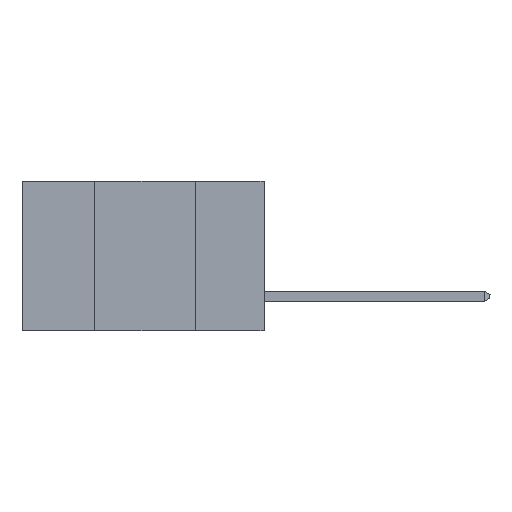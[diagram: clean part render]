
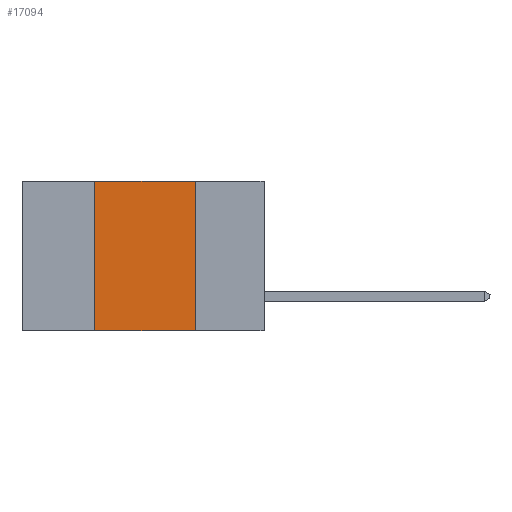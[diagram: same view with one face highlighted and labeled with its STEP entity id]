
A CAD part, left-side view. The second image highlights one B-rep face of the part: STEP entity #17094.
In plain terms, the highlighted planar face has unit normal (-1, 0, 0).
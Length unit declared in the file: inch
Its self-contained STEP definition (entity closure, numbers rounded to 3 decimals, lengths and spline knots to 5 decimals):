
#972 = VERTEX_POINT ( 'NONE', #8678 ) ;
#1638 = DIRECTION ( 'NONE',  ( 0., 0., -1. ) ) ;
#3787 = VECTOR ( 'NONE', #4854, 39.37008 ) ;
#4854 = DIRECTION ( 'NONE',  ( 0., -1., 0. ) ) ;
#5273 = EDGE_LOOP ( 'NONE', ( #5302, #8342, #9848, #22234 ) ) ;
#5302 = ORIENTED_EDGE ( 'NONE', *, *, #13556, .F. ) ;
#5391 = LINE ( 'NONE', #8872, #3787 ) ;
#5508 = LINE ( 'NONE', #22607, #10928 ) ;
#5584 = AXIS2_PLACEMENT_3D ( 'NONE', #26096, #13872, #1638 ) ;
#5923 = EDGE_CURVE ( 'NONE', #19945, #9236, #24880, .T. ) ;
#6390 = DIRECTION ( 'NONE',  ( 0., 0., 1. ) ) ;
#6781 = CARTESIAN_POINT ( 'NONE',  ( 0., 0.6, -0.37 ) ) ;
#8342 = ORIENTED_EDGE ( 'NONE', *, *, #11159, .F. ) ;
#8678 = CARTESIAN_POINT ( 'NONE',  ( 0., 0.42, 0. ) ) ;
#8872 = CARTESIAN_POINT ( 'NONE',  ( 0., 0.6, 0. ) ) ;
#9236 = VERTEX_POINT ( 'NONE', #25097 ) ;
#9724 = CARTESIAN_POINT ( 'NONE',  ( 0., 0.42, -0.37 ) ) ;
#9848 = ORIENTED_EDGE ( 'NONE', *, *, #15381, .F. ) ;
#9915 = CARTESIAN_POINT ( 'NONE',  ( 0., 0.17, 0. ) ) ;
#10037 = CARTESIAN_POINT ( 'NONE',  ( 0., 0.17, 0. ) ) ;
#10928 = VECTOR ( 'NONE', #6390, 39.37008 ) ;
#11159 = EDGE_CURVE ( 'NONE', #972, #19440, #5391, .T. ) ;
#11657 = VECTOR ( 'NONE', #24311, 39.37008 ) ;
#11822 = PLANE ( 'NONE',  #5584 ) ;
#13556 = EDGE_CURVE ( 'NONE', #19440, #9236, #16157, .T. ) ;
#13872 = DIRECTION ( 'NONE',  ( 1., 0., 0. ) ) ;
#15381 = EDGE_CURVE ( 'NONE', #19945, #972, #5508, .T. ) ;
#16157 = LINE ( 'NONE', #10037, #11657 ) ;
#17094 = ADVANCED_FACE ( 'NONE', ( #19145 ), #11822, .F. ) ;
#19145 = FACE_OUTER_BOUND ( 'NONE', #5273, .T. ) ;
#19440 = VERTEX_POINT ( 'NONE', #9915 ) ;
#19791 = VECTOR ( 'NONE', #25141, 39.37008 ) ;
#19945 = VERTEX_POINT ( 'NONE', #9724 ) ;
#22234 = ORIENTED_EDGE ( 'NONE', *, *, #5923, .T. ) ;
#22607 = CARTESIAN_POINT ( 'NONE',  ( 0., 0.42, 0. ) ) ;
#24311 = DIRECTION ( 'NONE',  ( 0., 0., -1. ) ) ;
#24880 = LINE ( 'NONE', #6781, #19791 ) ;
#25097 = CARTESIAN_POINT ( 'NONE',  ( 0., 0.17, -0.37 ) ) ;
#25141 = DIRECTION ( 'NONE',  ( 0., -1., 0. ) ) ;
#26096 = CARTESIAN_POINT ( 'NONE',  ( 0., 0.6, 0. ) ) ;
